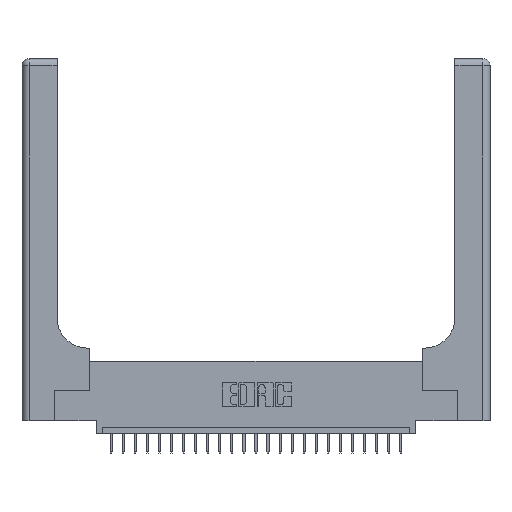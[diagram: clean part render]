
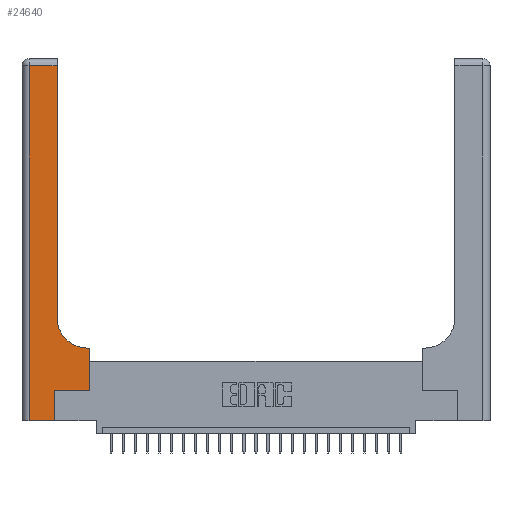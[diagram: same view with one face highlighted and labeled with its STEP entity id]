
A CAD part, top view. The second image highlights one B-rep face of the part: STEP entity #24640.
In plain terms, the highlighted planar face has unit normal (0, 0, 1).
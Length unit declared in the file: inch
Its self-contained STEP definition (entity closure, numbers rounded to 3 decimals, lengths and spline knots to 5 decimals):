
#289 = VERTEX_POINT ( 'NONE', #2328 ) ;
#398 = DIRECTION ( 'NONE',  ( 0., 1., 0. ) ) ;
#1157 = VECTOR ( 'NONE', #398, 39.37008 ) ;
#1209 = DIRECTION ( 'NONE',  ( 1., 0., 0. ) ) ;
#1796 = LINE ( 'NONE', #5211, #21357 ) ;
#1949 = CARTESIAN_POINT ( 'NONE',  ( 0.06, 2.94, 0.37 ) ) ;
#2152 = DIRECTION ( 'NONE',  ( 1., 0., 0. ) ) ;
#2328 = CARTESIAN_POINT ( 'NONE',  ( 0.5585, 0.6, 0.37 ) ) ;
#3752 = VECTOR ( 'NONE', #12168, 39.37008 ) ;
#4252 = DIRECTION ( 'NONE',  ( -1., 0., 0. ) ) ;
#4810 = ORIENTED_EDGE ( 'NONE', *, *, #7043, .T. ) ;
#5211 = CARTESIAN_POINT ( 'NONE',  ( 0.2915, 0.6, 0.37 ) ) ;
#5278 = CIRCLE ( 'NONE', #6703, 0.25 ) ;
#5395 = VERTEX_POINT ( 'NONE', #19061 ) ;
#5420 = EDGE_CURVE ( 'NONE', #10189, #10318, #22934, .T. ) ;
#5982 = VERTEX_POINT ( 'NONE', #6758 ) ;
#6046 = LINE ( 'NONE', #16596, #1157 ) ;
#6671 = ORIENTED_EDGE ( 'NONE', *, *, #5420, .T. ) ;
#6703 = AXIS2_PLACEMENT_3D ( 'NONE', #20132, #9693, #18013 ) ;
#6758 = CARTESIAN_POINT ( 'NONE',  ( 0.5415, 0.6, 0.37 ) ) ;
#7043 = EDGE_CURVE ( 'NONE', #11602, #289, #15507, .T. ) ;
#7479 = CARTESIAN_POINT ( 'NONE',  ( 0.2915, 2.94, 0.37 ) ) ;
#8110 = VECTOR ( 'NONE', #13575, 39.37008 ) ;
#8344 = VECTOR ( 'NONE', #4252, 39.37008 ) ;
#8858 = LINE ( 'NONE', #25722, #23849 ) ;
#8955 = ORIENTED_EDGE ( 'NONE', *, *, #22274, .T. ) ;
#9094 = VECTOR ( 'NONE', #10338, 39.37008 ) ;
#9588 = EDGE_CURVE ( 'NONE', #289, #5982, #1796, .T. ) ;
#9623 = FACE_OUTER_BOUND ( 'NONE', #12732, .T. ) ;
#9693 = DIRECTION ( 'NONE',  ( 0., 0., -1. ) ) ;
#10189 = VERTEX_POINT ( 'NONE', #17156 ) ;
#10318 = VERTEX_POINT ( 'NONE', #26113 ) ;
#10338 = DIRECTION ( 'NONE',  ( 0., 1., 0. ) ) ;
#10555 = CARTESIAN_POINT ( 'NONE',  ( 0.5585, 0.25, 0.37 ) ) ;
#10643 = LINE ( 'NONE', #23572, #8110 ) ;
#10759 = ORIENTED_EDGE ( 'NONE', *, *, #23737, .T. ) ;
#11026 = DIRECTION ( 'NONE',  ( -1., 0., 0. ) ) ;
#11602 = VERTEX_POINT ( 'NONE', #10555 ) ;
#11886 = VERTEX_POINT ( 'NONE', #1949 ) ;
#12168 = DIRECTION ( 'NONE',  ( 0., 1., 0. ) ) ;
#12732 = EDGE_LOOP ( 'NONE', ( #17387, #10759, #16212, #19427, #6671, #8955, #4810, #21461, #22060 ) ) ;
#12838 = EDGE_CURVE ( 'NONE', #11886, #5395, #10643, .T. ) ;
#13575 = DIRECTION ( 'NONE',  ( 0., -1., 0. ) ) ;
#13938 = VERTEX_POINT ( 'NONE', #7479 ) ;
#14286 = CARTESIAN_POINT ( 'NONE',  ( 0.5585, 0.25, 0.37 ) ) ;
#15059 = EDGE_CURVE ( 'NONE', #5395, #10189, #8858, .T. ) ;
#15507 = LINE ( 'NONE', #14286, #9094 ) ;
#16212 = ORIENTED_EDGE ( 'NONE', *, *, #12838, .T. ) ;
#16520 = CARTESIAN_POINT ( 'NONE',  ( 0., 2.94, 0.37 ) ) ;
#16596 = CARTESIAN_POINT ( 'NONE',  ( 0.2915, 3., 0.37 ) ) ;
#16640 = LINE ( 'NONE', #16520, #8344 ) ;
#17156 = CARTESIAN_POINT ( 'NONE',  ( 0.269, 0., 0.37 ) ) ;
#17212 = EDGE_CURVE ( 'NONE', #25648, #13938, #6046, .T. ) ;
#17353 = EDGE_CURVE ( 'NONE', #5982, #25648, #5278, .T. ) ;
#17387 = ORIENTED_EDGE ( 'NONE', *, *, #17212, .T. ) ;
#18013 = DIRECTION ( 'NONE',  ( 1., 0., 0. ) ) ;
#18468 = CARTESIAN_POINT ( 'NONE',  ( 0.269, 0.25, 0.37 ) ) ;
#19061 = CARTESIAN_POINT ( 'NONE',  ( 0.06, 0., 0.37 ) ) ;
#19091 = CARTESIAN_POINT ( 'NONE',  ( 0.2915, 0.85, 0.37 ) ) ;
#19323 = DIRECTION ( 'NONE',  ( 0., 0., -1. ) ) ;
#19427 = ORIENTED_EDGE ( 'NONE', *, *, #15059, .T. ) ;
#19489 = CARTESIAN_POINT ( 'NONE',  ( 0., 3., 0.37 ) ) ;
#20132 = CARTESIAN_POINT ( 'NONE',  ( 0.5415, 0.85, 0.37 ) ) ;
#20855 = LINE ( 'NONE', #18468, #22794 ) ;
#21357 = VECTOR ( 'NONE', #21911, 39.37008 ) ;
#21461 = ORIENTED_EDGE ( 'NONE', *, *, #9588, .T. ) ;
#21911 = DIRECTION ( 'NONE',  ( -1., 0., 0. ) ) ;
#22060 = ORIENTED_EDGE ( 'NONE', *, *, #17353, .T. ) ;
#22274 = EDGE_CURVE ( 'NONE', #10318, #11602, #20855, .T. ) ;
#22794 = VECTOR ( 'NONE', #2152, 39.37008 ) ;
#22934 = LINE ( 'NONE', #25888, #3752 ) ;
#23250 = PLANE ( 'NONE',  #23922 ) ;
#23572 = CARTESIAN_POINT ( 'NONE',  ( 0.06, 3., 0.37 ) ) ;
#23737 = EDGE_CURVE ( 'NONE', #13938, #11886, #16640, .T. ) ;
#23849 = VECTOR ( 'NONE', #1209, 39.37008 ) ;
#23922 = AXIS2_PLACEMENT_3D ( 'NONE', #19489, #19323, #11026 ) ;
#24640 = ADVANCED_FACE ( 'NONE', ( #9623 ), #23250, .F. ) ;
#25648 = VERTEX_POINT ( 'NONE', #19091 ) ;
#25722 = CARTESIAN_POINT ( 'NONE',  ( 0., 0., 0.37 ) ) ;
#25888 = CARTESIAN_POINT ( 'NONE',  ( 0.269, 0., 0.37 ) ) ;
#26113 = CARTESIAN_POINT ( 'NONE',  ( 0.269, 0.25, 0.37 ) ) ;
